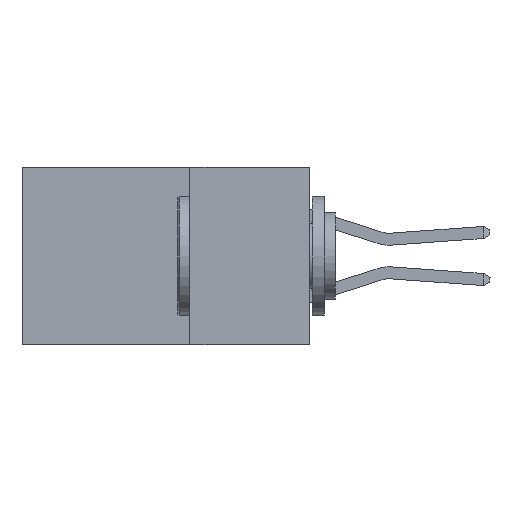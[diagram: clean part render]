
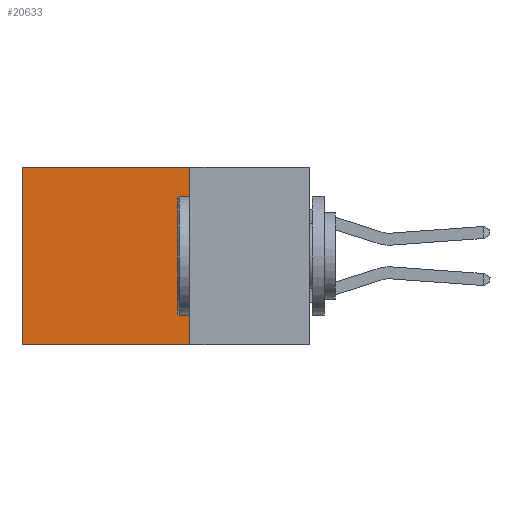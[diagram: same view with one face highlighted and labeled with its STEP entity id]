
A CAD part, left-side view. The second image highlights one B-rep face of the part: STEP entity #20633.
In plain terms, the highlighted planar face has unit normal (-1, 0, 0).
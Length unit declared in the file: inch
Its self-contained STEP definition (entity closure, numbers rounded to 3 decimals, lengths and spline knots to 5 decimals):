
#1238 = CARTESIAN_POINT ( 'NONE',  ( 0.2615, 0.6, -0.37 ) ) ;
#1459 = LINE ( 'NONE', #15682, #14295 ) ;
#1517 = PLANE ( 'NONE',  #7266 ) ;
#1552 = CARTESIAN_POINT ( 'NONE',  ( 0.2615, 0.6, -0.37 ) ) ;
#1892 = VECTOR ( 'NONE', #16374, 39.37008 ) ;
#2995 = VERTEX_POINT ( 'NONE', #16674 ) ;
#4781 = VERTEX_POINT ( 'NONE', #8531 ) ;
#4847 = VECTOR ( 'NONE', #17488, 39.37008 ) ;
#4934 = DIRECTION ( 'NONE',  ( 0., 0., -1. ) ) ;
#4939 = CARTESIAN_POINT ( 'NONE',  ( 0.2615, 0.25, -0.37 ) ) ;
#5376 = LINE ( 'NONE', #14161, #4847 ) ;
#6953 = VERTEX_POINT ( 'NONE', #1552 ) ;
#7266 = AXIS2_PLACEMENT_3D ( 'NONE', #21483, #14914, #4934 ) ;
#7406 = DIRECTION ( 'NONE',  ( 0., 1., 0. ) ) ;
#8482 = ORIENTED_EDGE ( 'NONE', *, *, #18647, .F. ) ;
#8531 = CARTESIAN_POINT ( 'NONE',  ( 0.2615, 0.6, 0. ) ) ;
#9512 = ORIENTED_EDGE ( 'NONE', *, *, #14586, .F. ) ;
#10829 = VECTOR ( 'NONE', #21329, 39.37008 ) ;
#13154 = EDGE_CURVE ( 'NONE', #2995, #4781, #1459, .T. ) ;
#14161 = CARTESIAN_POINT ( 'NONE',  ( 0.2615, 0.25, -0.37 ) ) ;
#14295 = VECTOR ( 'NONE', #7406, 39.37008 ) ;
#14586 = EDGE_CURVE ( 'NONE', #21227, #6953, #5376, .T. ) ;
#14914 = DIRECTION ( 'NONE',  ( 1., 0., 0. ) ) ;
#15682 = CARTESIAN_POINT ( 'NONE',  ( 0.2615, 0.25, 0. ) ) ;
#16087 = EDGE_CURVE ( 'NONE', #4781, #6953, #19609, .T. ) ;
#16184 = ORIENTED_EDGE ( 'NONE', *, *, #13154, .T. ) ;
#16374 = DIRECTION ( 'NONE',  ( 0., 0., -1. ) ) ;
#16674 = CARTESIAN_POINT ( 'NONE',  ( 0.2615, 0.25, 0. ) ) ;
#17364 = ORIENTED_EDGE ( 'NONE', *, *, #16087, .T. ) ;
#17488 = DIRECTION ( 'NONE',  ( 0., 1., 0. ) ) ;
#18647 = EDGE_CURVE ( 'NONE', #2995, #21227, #19600, .T. ) ;
#18706 = EDGE_LOOP ( 'NONE', ( #17364, #9512, #8482, #16184 ) ) ;
#19600 = LINE ( 'NONE', #20028, #10829 ) ;
#19609 = LINE ( 'NONE', #1238, #1892 ) ;
#19772 = FACE_OUTER_BOUND ( 'NONE', #18706, .T. ) ;
#20028 = CARTESIAN_POINT ( 'NONE',  ( 0.2615, 0.25, -0.37 ) ) ;
#20633 = ADVANCED_FACE ( 'NONE', ( #19772 ), #1517, .F. ) ;
#21227 = VERTEX_POINT ( 'NONE', #4939 ) ;
#21329 = DIRECTION ( 'NONE',  ( 0., 0., -1. ) ) ;
#21483 = CARTESIAN_POINT ( 'NONE',  ( 0.2615, 0.25, -0.37 ) ) ;
